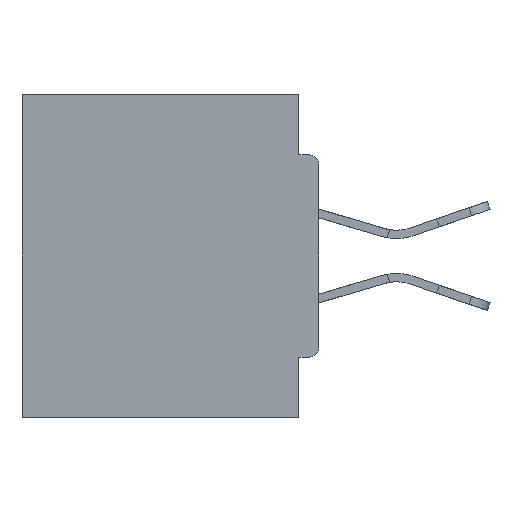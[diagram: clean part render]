
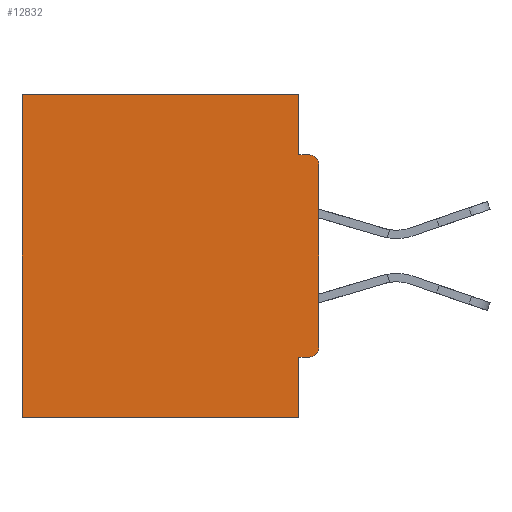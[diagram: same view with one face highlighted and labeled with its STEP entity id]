
A CAD part, left-side view. The second image highlights one B-rep face of the part: STEP entity #12832.
In plain terms, the highlighted planar face has unit normal (-1, 0, 0).
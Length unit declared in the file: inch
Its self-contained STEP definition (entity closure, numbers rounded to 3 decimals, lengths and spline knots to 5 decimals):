
#97 = AXIS2_PLACEMENT_3D ( 'NONE', #23016, #16504, #22734 ) ;
#280 = CARTESIAN_POINT ( 'NONE',  ( 0.298, 0.46, -0.5 ) ) ;
#341 = LINE ( 'NONE', #6111, #29737 ) ;
#663 = LINE ( 'NONE', #16507, #27543 ) ;
#1007 = VERTEX_POINT ( 'NONE', #31619 ) ;
#1166 = CIRCLE ( 'NONE', #22164, 0.015 ) ;
#1170 = VERTEX_POINT ( 'NONE', #280 ) ;
#2044 = LINE ( 'NONE', #23784, #27364 ) ;
#2267 = VECTOR ( 'NONE', #18668, 39.37008 ) ;
#3091 = LINE ( 'NONE', #22813, #22343 ) ;
#3483 = DIRECTION ( 'NONE',  ( 0., -1., 0. ) ) ;
#3644 = VERTEX_POINT ( 'NONE', #14714 ) ;
#3853 = VECTOR ( 'NONE', #20857, 39.37008 ) ;
#4402 = EDGE_CURVE ( 'NONE', #1007, #10879, #27691, .T. ) ;
#4998 = CARTESIAN_POINT ( 'NONE',  ( 0.298, 0., 0. ) ) ;
#5151 = DIRECTION ( 'NONE',  ( 1., 0., 0. ) ) ;
#5791 = CARTESIAN_POINT ( 'NONE',  ( 0.298, 0., 0. ) ) ;
#6111 = CARTESIAN_POINT ( 'NONE',  ( 0.298, 0.46, 0. ) ) ;
#6537 = DIRECTION ( 'NONE',  ( 0., 1., 0. ) ) ;
#8393 = PLANE ( 'NONE',  #33106 ) ;
#8915 = ORIENTED_EDGE ( 'NONE', *, *, #19623, .F. ) ;
#9684 = ORIENTED_EDGE ( 'NONE', *, *, #35612, .F. ) ;
#10879 = VERTEX_POINT ( 'NONE', #37763 ) ;
#10896 = VERTEX_POINT ( 'NONE', #19122 ) ;
#11114 = CARTESIAN_POINT ( 'NONE',  ( 0.298, 0.015, -0.3915 ) ) ;
#11236 = EDGE_CURVE ( 'NONE', #3644, #10896, #13395, .T. ) ;
#12285 = DIRECTION ( 'NONE',  ( 0., 0., -1. ) ) ;
#12809 = CARTESIAN_POINT ( 'NONE',  ( 0.298, 0.015, -0.4065 ) ) ;
#12832 = ADVANCED_FACE ( 'NONE', ( #19323 ), #8393, .F. ) ;
#13121 = EDGE_CURVE ( 'NONE', #10879, #1170, #3091, .T. ) ;
#13395 = LINE ( 'NONE', #5791, #2267 ) ;
#13538 = VERTEX_POINT ( 'NONE', #12809 ) ;
#14714 = CARTESIAN_POINT ( 'NONE',  ( 0.298, 0.031, 0. ) ) ;
#16504 = DIRECTION ( 'NONE',  ( -1., 0., 0. ) ) ;
#16507 = CARTESIAN_POINT ( 'NONE',  ( 0.298, 0., -0.0935 ) ) ;
#18498 = VECTOR ( 'NONE', #12285, 39.37008 ) ;
#18668 = DIRECTION ( 'NONE',  ( 0., 1., 0. ) ) ;
#19122 = CARTESIAN_POINT ( 'NONE',  ( 0.298, 0.46, 0. ) ) ;
#19323 = FACE_OUTER_BOUND ( 'NONE', #29908, .T. ) ;
#19623 = EDGE_CURVE ( 'NONE', #13538, #1007, #38442, .T. ) ;
#20132 = CIRCLE ( 'NONE', #97, 0.015 ) ;
#20857 = DIRECTION ( 'NONE',  ( 0., 0., -1. ) ) ;
#21203 = EDGE_CURVE ( 'NONE', #13538, #31944, #1166, .T. ) ;
#21737 = DIRECTION ( 'NONE',  ( 0., 1., 0. ) ) ;
#22164 = AXIS2_PLACEMENT_3D ( 'NONE', #11114, #40606, #33952 ) ;
#22343 = VECTOR ( 'NONE', #6537, 39.37008 ) ;
#22734 = DIRECTION ( 'NONE',  ( 0., 0., -1. ) ) ;
#22763 = EDGE_CURVE ( 'NONE', #31739, #31944, #29650, .T. ) ;
#22813 = CARTESIAN_POINT ( 'NONE',  ( 0.298, 0., -0.5 ) ) ;
#23016 = CARTESIAN_POINT ( 'NONE',  ( 0.298, 0.015, -0.1085 ) ) ;
#23049 = ORIENTED_EDGE ( 'NONE', *, *, #27793, .T. ) ;
#23784 = CARTESIAN_POINT ( 'NONE',  ( 0.298, 0.031, -0.5 ) ) ;
#24299 = CARTESIAN_POINT ( 'NONE',  ( 0.298, 0.015, -0.0935 ) ) ;
#26871 = EDGE_CURVE ( 'NONE', #31739, #40264, #20132, .T. ) ;
#27061 = ORIENTED_EDGE ( 'NONE', *, *, #4402, .F. ) ;
#27214 = VECTOR ( 'NONE', #21737, 39.37008 ) ;
#27364 = VECTOR ( 'NONE', #39825, 39.37008 ) ;
#27543 = VECTOR ( 'NONE', #3483, 39.37008 ) ;
#27691 = LINE ( 'NONE', #37201, #3853 ) ;
#27793 = EDGE_CURVE ( 'NONE', #10896, #1170, #341, .T. ) ;
#29650 = LINE ( 'NONE', #34865, #18498 ) ;
#29737 = VECTOR ( 'NONE', #35618, 39.37008 ) ;
#29908 = EDGE_LOOP ( 'NONE', ( #31363, #9684, #31203, #37459, #23049, #31513, #27061, #8915, #38943, #36349 ) ) ;
#31203 = ORIENTED_EDGE ( 'NONE', *, *, #33024, .F. ) ;
#31357 = DIRECTION ( 'NONE',  ( 0., 0., -1. ) ) ;
#31363 = ORIENTED_EDGE ( 'NONE', *, *, #26871, .T. ) ;
#31513 = ORIENTED_EDGE ( 'NONE', *, *, #13121, .F. ) ;
#31619 = CARTESIAN_POINT ( 'NONE',  ( 0.298, 0.031, -0.4065 ) ) ;
#31739 = VERTEX_POINT ( 'NONE', #41782 ) ;
#31944 = VERTEX_POINT ( 'NONE', #36677 ) ;
#33024 = EDGE_CURVE ( 'NONE', #3644, #34957, #2044, .T. ) ;
#33106 = AXIS2_PLACEMENT_3D ( 'NONE', #4998, #5151, #31357 ) ;
#33952 = DIRECTION ( 'NONE',  ( 0., 0., -1. ) ) ;
#34865 = CARTESIAN_POINT ( 'NONE',  ( 0.298, 0., 0. ) ) ;
#34957 = VERTEX_POINT ( 'NONE', #37195 ) ;
#35612 = EDGE_CURVE ( 'NONE', #34957, #40264, #663, .T. ) ;
#35618 = DIRECTION ( 'NONE',  ( 0., 0., -1. ) ) ;
#36349 = ORIENTED_EDGE ( 'NONE', *, *, #22763, .F. ) ;
#36677 = CARTESIAN_POINT ( 'NONE',  ( 0.298, 0., -0.3915 ) ) ;
#37195 = CARTESIAN_POINT ( 'NONE',  ( 0.298, 0.031, -0.0935 ) ) ;
#37201 = CARTESIAN_POINT ( 'NONE',  ( 0.298, 0.031, -0.5 ) ) ;
#37459 = ORIENTED_EDGE ( 'NONE', *, *, #11236, .T. ) ;
#37763 = CARTESIAN_POINT ( 'NONE',  ( 0.298, 0.031, -0.5 ) ) ;
#38442 = LINE ( 'NONE', #41715, #27214 ) ;
#38943 = ORIENTED_EDGE ( 'NONE', *, *, #21203, .T. ) ;
#39825 = DIRECTION ( 'NONE',  ( 0., 0., -1. ) ) ;
#40264 = VERTEX_POINT ( 'NONE', #24299 ) ;
#40606 = DIRECTION ( 'NONE',  ( -1., 0., 0. ) ) ;
#41715 = CARTESIAN_POINT ( 'NONE',  ( 0.298, 0., -0.4065 ) ) ;
#41782 = CARTESIAN_POINT ( 'NONE',  ( 0.298, 0., -0.1085 ) ) ;
